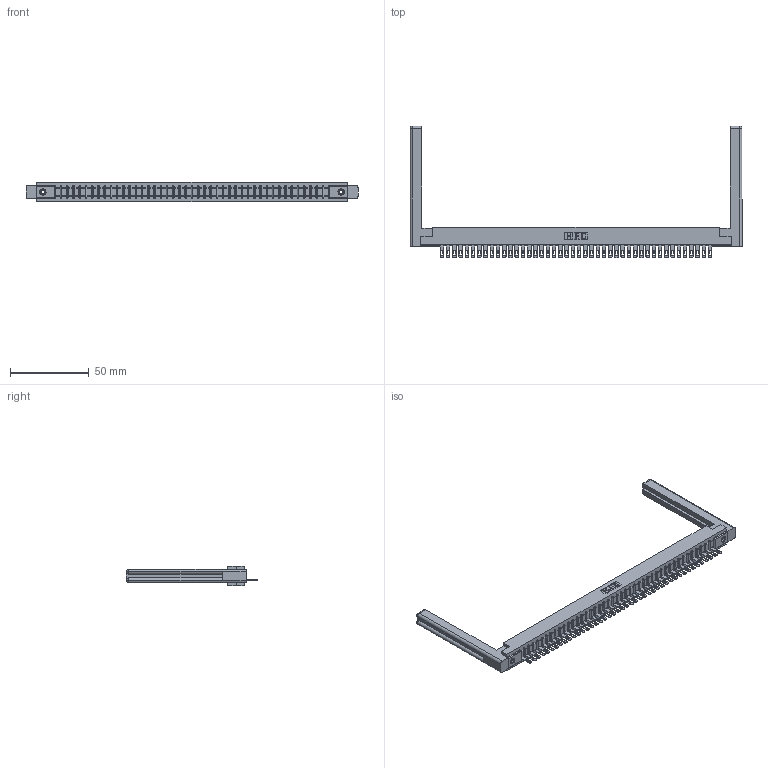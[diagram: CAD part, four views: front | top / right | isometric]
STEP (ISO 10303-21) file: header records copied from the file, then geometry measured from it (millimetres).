
FILE_DESCRIPTION (( 'STEP AP203' ), '1' );
FILE_NAME ('357-044-405-158.STEP', '2020-10-03T14:12:22', ( '' ), ( '' ), 'SwSTEP 2.0', 'SolidWorks 2020', '' );
FILE_SCHEMA (( 'CONFIG_CONTROL_DESIGN' ));
Length unit declared in the file: inch
Products named in the file (5): 345-250-001_345-250-001-102; 307-220-058; 307 Part_.156 Dia Mounting Holes; 357-044-405-158; 307-290-001_505
Assembly tree (49 placements, depth 2):
  357-044-405-158
    307 Part_.156 Dia Mounting Holes
    307-290-001_505  x44
    307-220-058  x2
    345-250-001_345-250-001-102  x2
Bounding box: 210.97 x 83.49 x 12.7 mm (x, y, z)
Volume: 29136.4 mm3; surface area: 28834.1 mm2
Topology: 49 solids, 49 shells, 2769 faces, 7805 edges, 5010 vertices
Faces by surface type: plane 1738, cylinder 917, sphere 90, torus 12, cone 12
Entity records: 40081 total; most frequent: CARTESIAN_POINT 6759, ORIENTED_EDGE 6684, DIRECTION 6534, EDGE_CURVE 3342, LINE 2560, VECTOR 2560, VERTEX_POINT 2158, AXIS2_PLACEMENT_3D 1987
